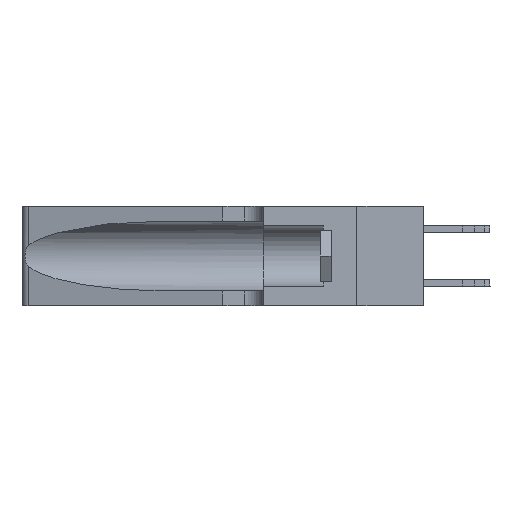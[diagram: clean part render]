
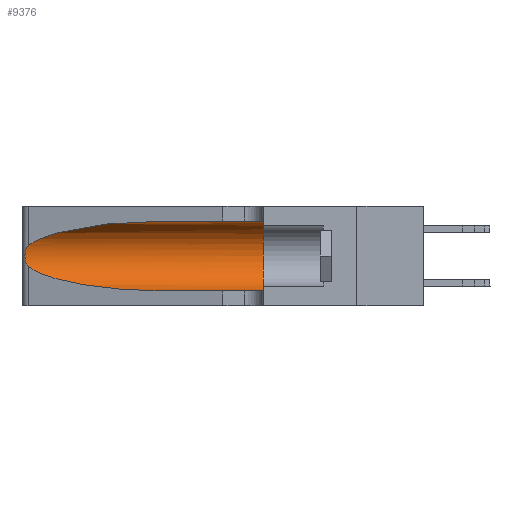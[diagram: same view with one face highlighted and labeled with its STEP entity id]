
A CAD part, left-side view. The second image highlights one B-rep face of the part: STEP entity #9376.
In plain terms, the highlighted cylindrical face has radius 3.308 mm (diameter 6.617 mm), a partial arc.
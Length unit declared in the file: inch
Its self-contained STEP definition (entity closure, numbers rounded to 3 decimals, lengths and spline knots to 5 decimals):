
#241 = VERTEX_POINT ( 'NONE', #10664 ) ;
#476 = CARTESIAN_POINT ( 'NONE',  ( 0.18966, 0.96281, 0.31525 ) ) ;
#1165 = CARTESIAN_POINT ( 'NONE',  ( 0.25555, 1.22993, 0.14849 ) ) ;
#2373 = VERTEX_POINT ( 'NONE', #2779 ) ;
#2685 = CARTESIAN_POINT ( 'NONE',  ( 0.1305, 0.72297, 0.31525 ) ) ;
#2779 = CARTESIAN_POINT ( 'NONE',  ( 0.1305, 0.35, 0.05475 ) ) ;
#2827 = CARTESIAN_POINT ( 'NONE',  ( 0.26075, 1.23896, 0.178 ) ) ;
#2910 = CARTESIAN_POINT ( 'NONE',  ( 0.1305, 0.35, 0.185 ) ) ;
#3027 = CARTESIAN_POINT ( 'NONE',  ( 0.26017, 1.23833, 0.17102 ) ) ;
#3147 = VERTEX_POINT ( 'NONE', #25796 ) ;
#3248 = VERTEX_POINT ( 'NONE', #27821 ) ;
#3316 = AXIS2_PLACEMENT_3D ( 'NONE', #17807, #13633, #13455 ) ;
#3456 = ORIENTED_EDGE ( 'NONE', *, *, #21156, .F. ) ;
#4850 = CARTESIAN_POINT ( 'NONE',  ( 0.25487, 1.22718, 0.22369 ) ) ;
#5209 = CARTESIAN_POINT ( 'NONE',  ( 0.18966, 0.96281, 0.05475 ) ) ;
#5412 = CARTESIAN_POINT ( 'NONE',  ( 0.25639, 1.23186, 0.15144 ) ) ;
#5589 = CARTESIAN_POINT ( 'NONE',  ( 0.1305, 0.72297, 0.05475 ) ) ;
#5808 = VECTOR ( 'NONE', #14717, 39.37008 ) ;
#5836 = EDGE_CURVE ( 'NONE', #3147, #21620, #24530, .T. ) ;
#7073 = CARTESIAN_POINT ( 'NONE',  ( 0.1305, 1.61858, 0.05475 ) ) ;
#8180 = CARTESIAN_POINT ( 'NONE',  ( 0.1305, 1.61858, 0.31525 ) ) ;
#9176 = DIRECTION ( 'NONE',  ( 0., 1., 0. ) ) ;
#9376 = ADVANCED_FACE ( 'NONE', ( #17608 ), #11732, .F. ) ;
#9610 = EDGE_CURVE ( 'NONE', #21620, #21220, #26425, .T. ) ;
#9756 = CARTESIAN_POINT ( 'NONE',  ( 0.25487, 1.22718, 0.14631 ) ) ;
#10664 = CARTESIAN_POINT ( 'NONE',  ( 0.1305, 0.35, 0.31525 ) ) ;
#11405 = DIRECTION ( 'NONE',  ( 0., -1., 0. ) ) ;
#11556 = ORIENTED_EDGE ( 'NONE', *, *, #15580, .T. ) ;
#11575 = CARTESIAN_POINT ( 'NONE',  ( 0.25639, 1.23184, 0.21858 ) ) ;
#11732 = CYLINDRICAL_SURFACE ( 'NONE', #3316, 0.13025 ) ;
#12053 = CARTESIAN_POINT ( 'NONE',  ( 0.25789, 1.23486, 0.15765 ) ) ;
#12328 = ORIENTED_EDGE ( 'NONE', *, *, #25197, .F. ) ;
#13419 = LINE ( 'NONE', #7073, #13772 ) ;
#13455 = DIRECTION ( 'NONE',  ( 0., 0., -1. ) ) ;
#13633 = DIRECTION ( 'NONE',  ( 0., -1., 0. ) ) ;
#13772 = VECTOR ( 'NONE', #11405, 39.37008 ) ;
#13781 = CARTESIAN_POINT ( 'NONE',  ( 0.26075, 1.23896, 0.19203 ) ) ;
#13873 = CARTESIAN_POINT ( 'NONE',  ( 0.25854, 1.2359, 0.20912 ) ) ;
#14344 = CARTESIAN_POINT ( 'NONE',  ( 0.25487, 1.22718, 0.14631 ) ) ;
#14717 = DIRECTION ( 'NONE',  ( 0., -1., 0. ) ) ;
#15580 = EDGE_CURVE ( 'NONE', #21220, #2373, #13419, .T. ) ;
#16015 = CARTESIAN_POINT ( 'NONE',  ( 0.25555, 1.22994, 0.2215 ) ) ;
#17608 = FACE_OUTER_BOUND ( 'NONE', #18330, .T. ) ;
#17807 = CARTESIAN_POINT ( 'NONE',  ( 0.1305, 1.61858, 0.185 ) ) ;
#18330 = EDGE_LOOP ( 'NONE', ( #26322, #19990, #27681, #11556, #12328, #3456 ) ) ;
#19990 = ORIENTED_EDGE ( 'NONE', *, *, #5836, .T. ) ;
#20258 = DIRECTION ( 'NONE',  ( 0., 0., 1. ) ) ;
#20272 = CARTESIAN_POINT ( 'NONE',  ( 0.25787, 1.23484, 0.2124 ) ) ;
#20414 = CARTESIAN_POINT ( 'NONE',  ( 0.25487, 1.22718, 0.22369 ) ) ;
#20604 = CARTESIAN_POINT ( 'NONE',  ( 0.2373, 1.15595, 0.28018 ) ) ;
#20735 = CARTESIAN_POINT ( 'NONE',  ( 0.2373, 1.15595, 0.08982 ) ) ;
#21156 = EDGE_CURVE ( 'NONE', #3248, #241, #24125, .T. ) ;
#21220 = VERTEX_POINT ( 'NONE', #25754 ) ;
#21620 = VERTEX_POINT ( 'NONE', #27193 ) ;
#21807 =( BOUNDED_CURVE ( )  B_SPLINE_CURVE ( 3, ( #2685, #476, #20604, #20414 ),
 .UNSPECIFIED., .F., .F. ) 
 B_SPLINE_CURVE_WITH_KNOTS ( ( 4, 4 ),
 ( 1.5708, 2.84003 ),
 .UNSPECIFIED. ) 
 CURVE ( )  GEOMETRIC_REPRESENTATION_ITEM ( )  RATIONAL_B_SPLINE_CURVE ( ( 1., 0.87, 0.87, 1. ) ) 
 REPRESENTATION_ITEM ( '' )  );
#21884 = AXIS2_PLACEMENT_3D ( 'NONE', #2910, #9176, #20258 ) ;
#22517 = CARTESIAN_POINT ( 'NONE',  ( 0.26018, 1.23835, 0.19895 ) ) ;
#22903 = CARTESIAN_POINT ( 'NONE',  ( 0.25856, 1.23593, 0.16098 ) ) ;
#24125 = LINE ( 'NONE', #8180, #5808 ) ;
#24530 = B_SPLINE_CURVE_WITH_KNOTS ( 'NONE', 3,
 ( #4850, #16015, #11575, #20272, #13873, #22517, #13781, #2827, #3027, #22903, #12053, #5412, #1165, #9756 ),
 .UNSPECIFIED., .F., .F.,
 ( 4, 2, 2, 2, 2, 2, 4 ),
 ( 0., 0.00027, 0.00053, 0.00107, 0.0016, 0.00187, 0.00214 ),
 .UNSPECIFIED. ) ;
#25197 = EDGE_CURVE ( 'NONE', #241, #2373, #27685, .T. ) ;
#25754 = CARTESIAN_POINT ( 'NONE',  ( 0.1305, 0.72297, 0.05475 ) ) ;
#25796 = CARTESIAN_POINT ( 'NONE',  ( 0.25487, 1.22718, 0.22369 ) ) ;
#25893 = EDGE_CURVE ( 'NONE', #3248, #3147, #21807, .T. ) ;
#26322 = ORIENTED_EDGE ( 'NONE', *, *, #25893, .T. ) ;
#26425 =( BOUNDED_CURVE ( )  B_SPLINE_CURVE ( 3, ( #14344, #20735, #5209, #5589 ),
 .UNSPECIFIED., .F., .F. ) 
 B_SPLINE_CURVE_WITH_KNOTS ( ( 4, 4 ),
 ( 3.44316, 4.71239 ),
 .UNSPECIFIED. ) 
 CURVE ( )  GEOMETRIC_REPRESENTATION_ITEM ( )  RATIONAL_B_SPLINE_CURVE ( ( 1., 0.87, 0.87, 1. ) ) 
 REPRESENTATION_ITEM ( '' )  );
#27193 = CARTESIAN_POINT ( 'NONE',  ( 0.25487, 1.22718, 0.14631 ) ) ;
#27681 = ORIENTED_EDGE ( 'NONE', *, *, #9610, .T. ) ;
#27685 = CIRCLE ( 'NONE', #21884, 0.13025 ) ;
#27821 = CARTESIAN_POINT ( 'NONE',  ( 0.1305, 0.72297, 0.31525 ) ) ;
